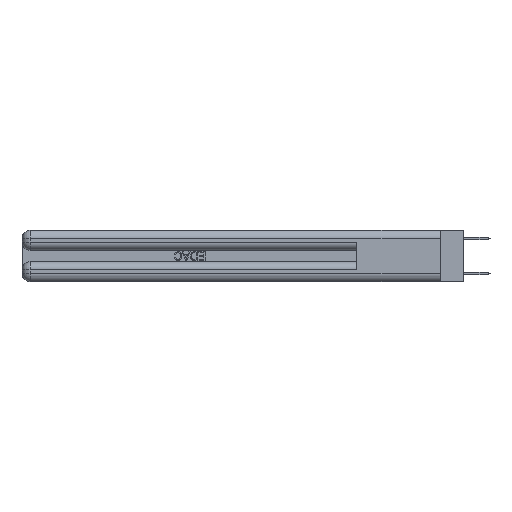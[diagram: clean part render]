
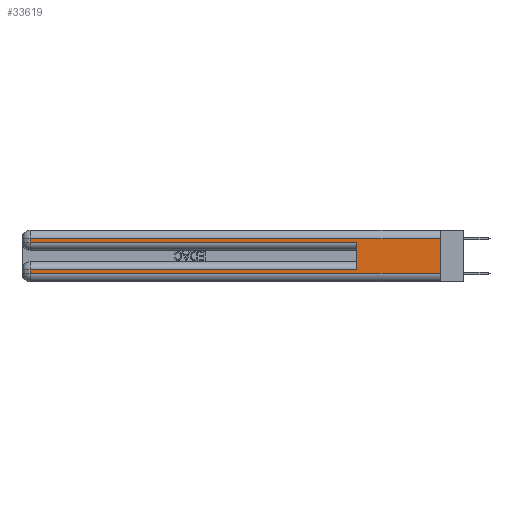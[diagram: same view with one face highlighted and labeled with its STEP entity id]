
A CAD part, left-side view. The second image highlights one B-rep face of the part: STEP entity #33619.
In plain terms, the highlighted planar face has unit normal (-1, 0, 0).
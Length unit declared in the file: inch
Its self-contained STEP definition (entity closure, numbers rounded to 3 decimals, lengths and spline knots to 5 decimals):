
#33 = LINE ( 'NONE', #10622, #26735 ) ;
#980 = CARTESIAN_POINT ( 'NONE',  ( 0., 0., 0.085 ) ) ;
#1031 = DIRECTION ( 'NONE',  ( 1., 0., 0. ) ) ;
#2490 = VERTEX_POINT ( 'NONE', #24475 ) ;
#2588 = CARTESIAN_POINT ( 'NONE',  ( 0., 0.6, 0.085 ) ) ;
#4425 = VECTOR ( 'NONE', #6897, 39.37008 ) ;
#5640 = EDGE_CURVE ( 'NONE', #6316, #9553, #10920, .T. ) ;
#6078 = DIRECTION ( 'NONE',  ( 0., 0., -1. ) ) ;
#6316 = VERTEX_POINT ( 'NONE', #33302 ) ;
#6341 = EDGE_CURVE ( 'NONE', #33874, #6316, #24730, .T. ) ;
#6348 = VERTEX_POINT ( 'NONE', #14322 ) ;
#6897 = DIRECTION ( 'NONE',  ( 0., 0., 1. ) ) ;
#7358 = DIRECTION ( 'NONE',  ( 0., 0., -1. ) ) ;
#8184 = DIRECTION ( 'NONE',  ( 0., 1., 0. ) ) ;
#9021 = DIRECTION ( 'NONE',  ( 0., 0., -1. ) ) ;
#9143 = CARTESIAN_POINT ( 'NONE',  ( 0., 0., 0.285 ) ) ;
#9553 = VERTEX_POINT ( 'NONE', #25059 ) ;
#9956 = LINE ( 'NONE', #20531, #30821 ) ;
#10422 = EDGE_CURVE ( 'NONE', #33874, #30841, #20239, .T. ) ;
#10622 = CARTESIAN_POINT ( 'NONE',  ( 0., 0., 0.31 ) ) ;
#10920 = LINE ( 'NONE', #24101, #31985 ) ;
#11504 = EDGE_CURVE ( 'NONE', #11645, #30841, #14503, .T. ) ;
#11645 = VERTEX_POINT ( 'NONE', #11743 ) ;
#11743 = CARTESIAN_POINT ( 'NONE',  ( 0., 2.94, 0.285 ) ) ;
#12377 = CARTESIAN_POINT ( 'NONE',  ( 0., 0., 0.37 ) ) ;
#13619 = CARTESIAN_POINT ( 'NONE',  ( 0., 0., 0.06 ) ) ;
#13711 = CARTESIAN_POINT ( 'NONE',  ( 0., 0.6, 0.285 ) ) ;
#14322 = CARTESIAN_POINT ( 'NONE',  ( 0., 2.94, 0.31 ) ) ;
#14503 = LINE ( 'NONE', #9143, #18875 ) ;
#15223 = CARTESIAN_POINT ( 'NONE',  ( 0., 0., 0.31 ) ) ;
#16072 = LINE ( 'NONE', #13619, #21293 ) ;
#16664 = FACE_OUTER_BOUND ( 'NONE', #21858, .T. ) ;
#17003 = CARTESIAN_POINT ( 'NONE',  ( 0., 0., 0.37 ) ) ;
#18875 = VECTOR ( 'NONE', #28077, 39.37008 ) ;
#19778 = AXIS2_PLACEMENT_3D ( 'NONE', #17003, #1031, #9021 ) ;
#20045 = EDGE_CURVE ( 'NONE', #20833, #6348, #33, .T. ) ;
#20155 = ORIENTED_EDGE ( 'NONE', *, *, #5640, .T. ) ;
#20239 = LINE ( 'NONE', #28585, #4425 ) ;
#20356 = LINE ( 'NONE', #12377, #31384 ) ;
#20531 = CARTESIAN_POINT ( 'NONE',  ( 0., 2.94, 0.37 ) ) ;
#20833 = VERTEX_POINT ( 'NONE', #15223 ) ;
#21127 = ORIENTED_EDGE ( 'NONE', *, *, #6341, .T. ) ;
#21293 = VECTOR ( 'NONE', #24548, 39.37008 ) ;
#21858 = EDGE_LOOP ( 'NONE', ( #25113, #26402, #33790, #29730, #32046, #21127, #20155, #24499 ) ) ;
#21973 = VECTOR ( 'NONE', #22126, 39.37008 ) ;
#22126 = DIRECTION ( 'NONE',  ( 0., 1., 0. ) ) ;
#24101 = CARTESIAN_POINT ( 'NONE',  ( 0., 2.94, 0.37 ) ) ;
#24475 = CARTESIAN_POINT ( 'NONE',  ( 0., 0., 0.06 ) ) ;
#24499 = ORIENTED_EDGE ( 'NONE', *, *, #25122, .T. ) ;
#24548 = DIRECTION ( 'NONE',  ( 0., -1., 0. ) ) ;
#24730 = LINE ( 'NONE', #980, #21973 ) ;
#24785 = PLANE ( 'NONE',  #19778 ) ;
#25059 = CARTESIAN_POINT ( 'NONE',  ( 0., 2.94, 0.06 ) ) ;
#25113 = ORIENTED_EDGE ( 'NONE', *, *, #25889, .F. ) ;
#25122 = EDGE_CURVE ( 'NONE', #9553, #2490, #16072, .T. ) ;
#25889 = EDGE_CURVE ( 'NONE', #20833, #2490, #20356, .T. ) ;
#25906 = EDGE_CURVE ( 'NONE', #6348, #11645, #9956, .T. ) ;
#26402 = ORIENTED_EDGE ( 'NONE', *, *, #20045, .T. ) ;
#26735 = VECTOR ( 'NONE', #8184, 39.37008 ) ;
#28077 = DIRECTION ( 'NONE',  ( 0., -1., 0. ) ) ;
#28585 = CARTESIAN_POINT ( 'NONE',  ( 0., 0.6, 0.145 ) ) ;
#29730 = ORIENTED_EDGE ( 'NONE', *, *, #11504, .T. ) ;
#30821 = VECTOR ( 'NONE', #7358, 39.37008 ) ;
#30841 = VERTEX_POINT ( 'NONE', #13711 ) ;
#30982 = DIRECTION ( 'NONE',  ( 0., 0., -1. ) ) ;
#31384 = VECTOR ( 'NONE', #30982, 39.37008 ) ;
#31985 = VECTOR ( 'NONE', #6078, 39.37008 ) ;
#32046 = ORIENTED_EDGE ( 'NONE', *, *, #10422, .F. ) ;
#33302 = CARTESIAN_POINT ( 'NONE',  ( 0., 2.94, 0.085 ) ) ;
#33619 = ADVANCED_FACE ( 'NONE', ( #16664 ), #24785, .F. ) ;
#33790 = ORIENTED_EDGE ( 'NONE', *, *, #25906, .T. ) ;
#33874 = VERTEX_POINT ( 'NONE', #2588 ) ;
